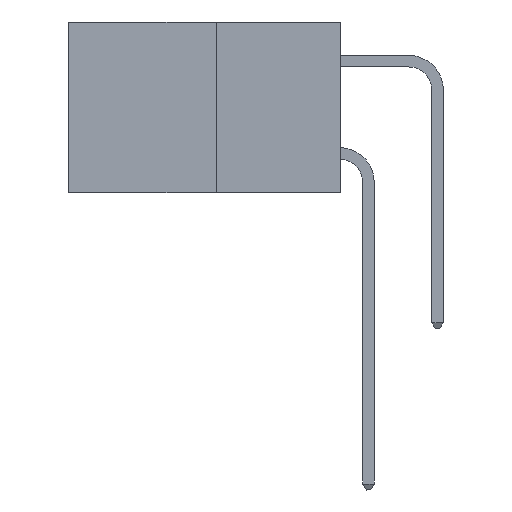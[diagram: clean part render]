
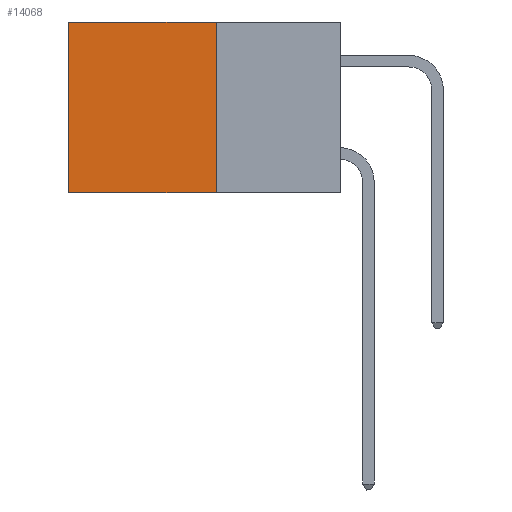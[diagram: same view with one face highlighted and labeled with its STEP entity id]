
A CAD part, left-side view. The second image highlights one B-rep face of the part: STEP entity #14068.
In plain terms, the highlighted planar face has unit normal (-1, 0, 0).
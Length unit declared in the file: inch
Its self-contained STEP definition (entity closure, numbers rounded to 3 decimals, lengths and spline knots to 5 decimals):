
#326 = PLANE ( 'NONE',  #2309 ) ;
#507 = VERTEX_POINT ( 'NONE', #3327 ) ;
#985 = ORIENTED_EDGE ( 'NONE', *, *, #1018, .F. ) ;
#1018 = EDGE_CURVE ( 'NONE', #507, #3009, #8621, .T. ) ;
#1210 = EDGE_CURVE ( 'NONE', #13810, #507, #7097, .T. ) ;
#1331 = ORIENTED_EDGE ( 'NONE', *, *, #12850, .T. ) ;
#1368 = ORIENTED_EDGE ( 'NONE', *, *, #11482, .T. ) ;
#1384 = ORIENTED_EDGE ( 'NONE', *, *, #1210, .F. ) ;
#2020 = DIRECTION ( 'NONE',  ( 0., 1., 0. ) ) ;
#2045 = CARTESIAN_POINT ( 'NONE',  ( 0.277, 0.27, 0. ) ) ;
#2309 = AXIS2_PLACEMENT_3D ( 'NONE', #10427, #3015, #11593 ) ;
#3009 = VERTEX_POINT ( 'NONE', #9261 ) ;
#3015 = DIRECTION ( 'NONE',  ( 1., 0., 0. ) ) ;
#3327 = CARTESIAN_POINT ( 'NONE',  ( 0.277, 0.27, -0.37 ) ) ;
#4025 = VECTOR ( 'NONE', #6957, 39.37008 ) ;
#5349 = VECTOR ( 'NONE', #11880, 39.37008 ) ;
#5715 = CARTESIAN_POINT ( 'NONE',  ( 0.277, 0.59, -0.37 ) ) ;
#5724 = EDGE_LOOP ( 'NONE', ( #1331, #985, #1384, #1368 ) ) ;
#6715 = FACE_OUTER_BOUND ( 'NONE', #5724, .T. ) ;
#6957 = DIRECTION ( 'NONE',  ( 0., 0., -1. ) ) ;
#6960 = LINE ( 'NONE', #2045, #12933 ) ;
#7097 = LINE ( 'NONE', #11824, #13049 ) ;
#8621 = LINE ( 'NONE', #14516, #5349 ) ;
#8847 = DIRECTION ( 'NONE',  ( 0., 0., -1. ) ) ;
#9261 = CARTESIAN_POINT ( 'NONE',  ( 0.277, 0.59, -0.37 ) ) ;
#10427 = CARTESIAN_POINT ( 'NONE',  ( 0.277, 0.27, -0.37 ) ) ;
#11482 = EDGE_CURVE ( 'NONE', #13810, #15144, #6960, .T. ) ;
#11593 = DIRECTION ( 'NONE',  ( 0., 0., -1. ) ) ;
#11824 = CARTESIAN_POINT ( 'NONE',  ( 0.277, 0.27, -0.37 ) ) ;
#11880 = DIRECTION ( 'NONE',  ( 0., 1., 0. ) ) ;
#12850 = EDGE_CURVE ( 'NONE', #15144, #3009, #13643, .T. ) ;
#12933 = VECTOR ( 'NONE', #2020, 39.37008 ) ;
#13049 = VECTOR ( 'NONE', #8847, 39.37008 ) ;
#13643 = LINE ( 'NONE', #5715, #4025 ) ;
#13810 = VERTEX_POINT ( 'NONE', #14600 ) ;
#14068 = ADVANCED_FACE ( 'NONE', ( #6715 ), #326, .F. ) ;
#14499 = CARTESIAN_POINT ( 'NONE',  ( 0.277, 0.59, 0. ) ) ;
#14516 = CARTESIAN_POINT ( 'NONE',  ( 0.277, 0.27, -0.37 ) ) ;
#14600 = CARTESIAN_POINT ( 'NONE',  ( 0.277, 0.27, 0. ) ) ;
#15144 = VERTEX_POINT ( 'NONE', #14499 ) ;
